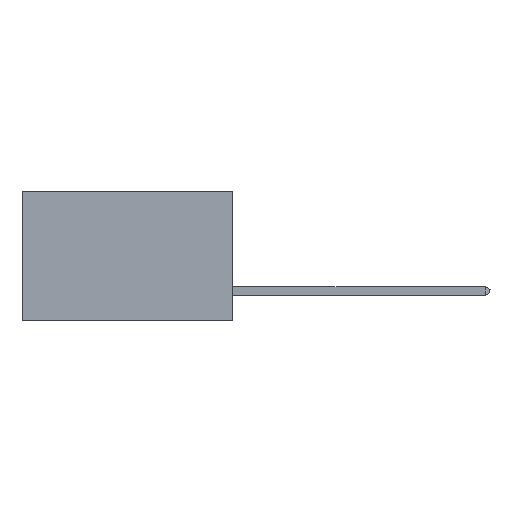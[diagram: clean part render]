
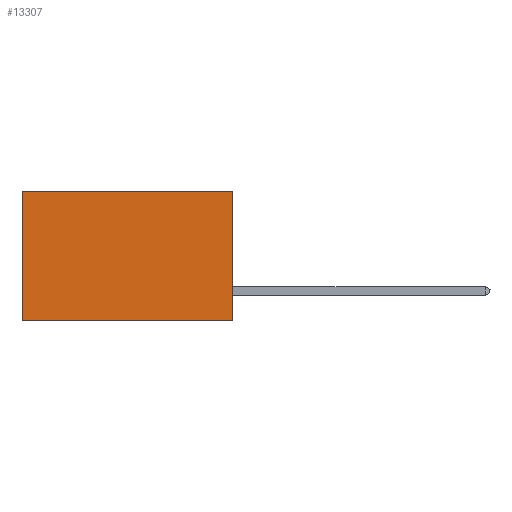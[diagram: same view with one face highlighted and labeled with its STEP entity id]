
A CAD part, left-side view. The second image highlights one B-rep face of the part: STEP entity #13307.
In plain terms, the highlighted planar face has unit normal (-1, 0, 0).
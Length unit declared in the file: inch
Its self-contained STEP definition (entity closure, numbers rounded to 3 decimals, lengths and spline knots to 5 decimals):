
#1718 = DIRECTION ( 'NONE',  ( 0., 0., -1. ) ) ;
#1862 = CARTESIAN_POINT ( 'NONE',  ( 0.2875, 0., 0. ) ) ;
#1926 = EDGE_CURVE ( 'NONE', #22166, #30756, #39800, .T. ) ;
#2012 = AXIS2_PLACEMENT_3D ( 'NONE', #1862, #32580, #1718 ) ;
#2583 = CARTESIAN_POINT ( 'NONE',  ( 0.2875, 0.6, 0. ) ) ;
#3360 = VERTEX_POINT ( 'NONE', #8863 ) ;
#3994 = FACE_OUTER_BOUND ( 'NONE', #12808, .T. ) ;
#4465 = CARTESIAN_POINT ( 'NONE',  ( 0.2875, 0., 0. ) ) ;
#5860 = VECTOR ( 'NONE', #12818, 39.37008 ) ;
#8393 = CARTESIAN_POINT ( 'NONE',  ( 0.2875, 0., -0.37 ) ) ;
#8863 = CARTESIAN_POINT ( 'NONE',  ( 0.2875, 0., -0.37 ) ) ;
#10017 = VECTOR ( 'NONE', #11579, 39.37008 ) ;
#10935 = ORIENTED_EDGE ( 'NONE', *, *, #1926, .T. ) ;
#10984 = PLANE ( 'NONE',  #2012 ) ;
#11100 = CARTESIAN_POINT ( 'NONE',  ( 0.2875, 0.6, 0. ) ) ;
#11324 = CARTESIAN_POINT ( 'NONE',  ( 0.2875, 0.6, -0.37 ) ) ;
#11362 = EDGE_CURVE ( 'NONE', #3360, #23466, #38187, .T. ) ;
#11579 = DIRECTION ( 'NONE',  ( 0., 1., 0. ) ) ;
#12808 = EDGE_LOOP ( 'NONE', ( #26384, #28413, #13419, #10935 ) ) ;
#12818 = DIRECTION ( 'NONE',  ( 0., 0., -1. ) ) ;
#13307 = ADVANCED_FACE ( 'NONE', ( #3994 ), #10984, .F. ) ;
#13419 = ORIENTED_EDGE ( 'NONE', *, *, #36559, .F. ) ;
#14079 = DIRECTION ( 'NONE',  ( 0., 0., -1. ) ) ;
#14665 = VECTOR ( 'NONE', #35807, 39.37008 ) ;
#21232 = EDGE_CURVE ( 'NONE', #30756, #23466, #28401, .T. ) ;
#22166 = VERTEX_POINT ( 'NONE', #4465 ) ;
#23466 = VERTEX_POINT ( 'NONE', #11324 ) ;
#23590 = VECTOR ( 'NONE', #14079, 39.37008 ) ;
#24975 = CARTESIAN_POINT ( 'NONE',  ( 0.2875, 0., 0. ) ) ;
#26384 = ORIENTED_EDGE ( 'NONE', *, *, #21232, .T. ) ;
#28401 = LINE ( 'NONE', #11100, #23590 ) ;
#28413 = ORIENTED_EDGE ( 'NONE', *, *, #11362, .F. ) ;
#30314 = LINE ( 'NONE', #24975, #5860 ) ;
#30756 = VERTEX_POINT ( 'NONE', #2583 ) ;
#32580 = DIRECTION ( 'NONE',  ( 1., 0., 0. ) ) ;
#35807 = DIRECTION ( 'NONE',  ( 0., 1., 0. ) ) ;
#36559 = EDGE_CURVE ( 'NONE', #22166, #3360, #30314, .T. ) ;
#38187 = LINE ( 'NONE', #8393, #14665 ) ;
#39504 = CARTESIAN_POINT ( 'NONE',  ( 0.2875, 0., 0. ) ) ;
#39800 = LINE ( 'NONE', #39504, #10017 ) ;
